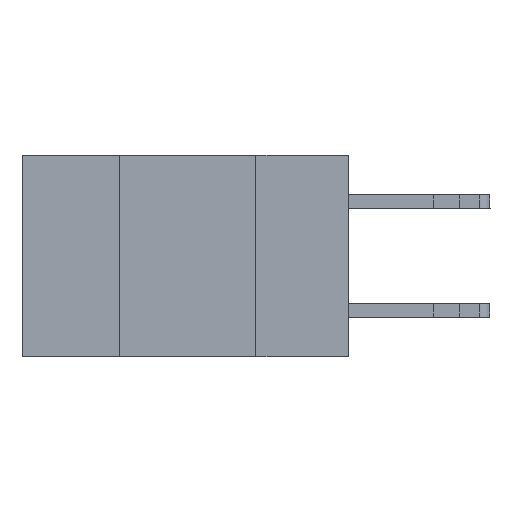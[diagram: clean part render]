
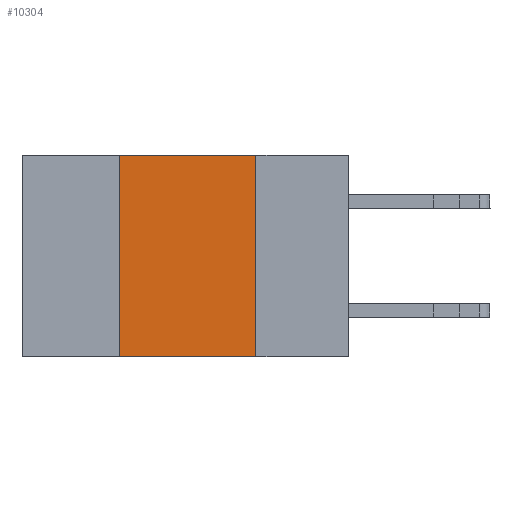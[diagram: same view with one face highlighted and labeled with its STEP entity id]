
A CAD part, left-side view. The second image highlights one B-rep face of the part: STEP entity #10304.
In plain terms, the highlighted planar face has unit normal (-1, 0, 0).
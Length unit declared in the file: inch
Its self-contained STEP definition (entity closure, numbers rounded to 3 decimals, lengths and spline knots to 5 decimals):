
#1020 = ORIENTED_EDGE ( 'NONE', *, *, #2344, .F. ) ;
#1540 = LINE ( 'NONE', #5082, #10519 ) ;
#1573 = CARTESIAN_POINT ( 'NONE',  ( 0., 0.17, -0.37 ) ) ;
#1574 = EDGE_CURVE ( 'NONE', #1942, #7276, #7054, .T. ) ;
#1784 = VECTOR ( 'NONE', #6008, 39.37008 ) ;
#1942 = VERTEX_POINT ( 'NONE', #3548 ) ;
#1967 = LINE ( 'NONE', #9645, #7745 ) ;
#2344 = EDGE_CURVE ( 'NONE', #7276, #2501, #12240, .T. ) ;
#2501 = VERTEX_POINT ( 'NONE', #4133 ) ;
#2749 = CARTESIAN_POINT ( 'NONE',  ( 0., 0.42, 0. ) ) ;
#3128 = FACE_OUTER_BOUND ( 'NONE', #13146, .T. ) ;
#3548 = CARTESIAN_POINT ( 'NONE',  ( 0., 0.42, -0.37 ) ) ;
#3794 = ORIENTED_EDGE ( 'NONE', *, *, #1574, .F. ) ;
#4133 = CARTESIAN_POINT ( 'NONE',  ( 0., 0.17, 0. ) ) ;
#5082 = CARTESIAN_POINT ( 'NONE',  ( 0., 0.17, 0. ) ) ;
#5281 = PLANE ( 'NONE',  #10533 ) ;
#5481 = CARTESIAN_POINT ( 'NONE',  ( 0., 0.6, 0. ) ) ;
#5995 = ORIENTED_EDGE ( 'NONE', *, *, #9602, .F. ) ;
#6008 = DIRECTION ( 'NONE',  ( 0., 0., 1. ) ) ;
#7054 = LINE ( 'NONE', #2749, #1784 ) ;
#7148 = DIRECTION ( 'NONE',  ( 0., 0., -1. ) ) ;
#7276 = VERTEX_POINT ( 'NONE', #13288 ) ;
#7745 = VECTOR ( 'NONE', #10790, 39.37008 ) ;
#8734 = DIRECTION ( 'NONE',  ( 0., -1., 0. ) ) ;
#9157 = VECTOR ( 'NONE', #8734, 39.37008 ) ;
#9602 = EDGE_CURVE ( 'NONE', #2501, #13026, #1540, .T. ) ;
#9645 = CARTESIAN_POINT ( 'NONE',  ( 0., 0.6, -0.37 ) ) ;
#9777 = DIRECTION ( 'NONE',  ( 1., 0., 0. ) ) ;
#10304 = ADVANCED_FACE ( 'NONE', ( #3128 ), #5281, .F. ) ;
#10519 = VECTOR ( 'NONE', #7148, 39.37008 ) ;
#10533 = AXIS2_PLACEMENT_3D ( 'NONE', #14163, #9777, #12043 ) ;
#10790 = DIRECTION ( 'NONE',  ( 0., -1., 0. ) ) ;
#10850 = EDGE_CURVE ( 'NONE', #1942, #13026, #1967, .T. ) ;
#11708 = ORIENTED_EDGE ( 'NONE', *, *, #10850, .T. ) ;
#12043 = DIRECTION ( 'NONE',  ( 0., 0., -1. ) ) ;
#12240 = LINE ( 'NONE', #5481, #9157 ) ;
#13026 = VERTEX_POINT ( 'NONE', #1573 ) ;
#13146 = EDGE_LOOP ( 'NONE', ( #5995, #1020, #3794, #11708 ) ) ;
#13288 = CARTESIAN_POINT ( 'NONE',  ( 0., 0.42, 0. ) ) ;
#14163 = CARTESIAN_POINT ( 'NONE',  ( 0., 0.6, 0. ) ) ;
